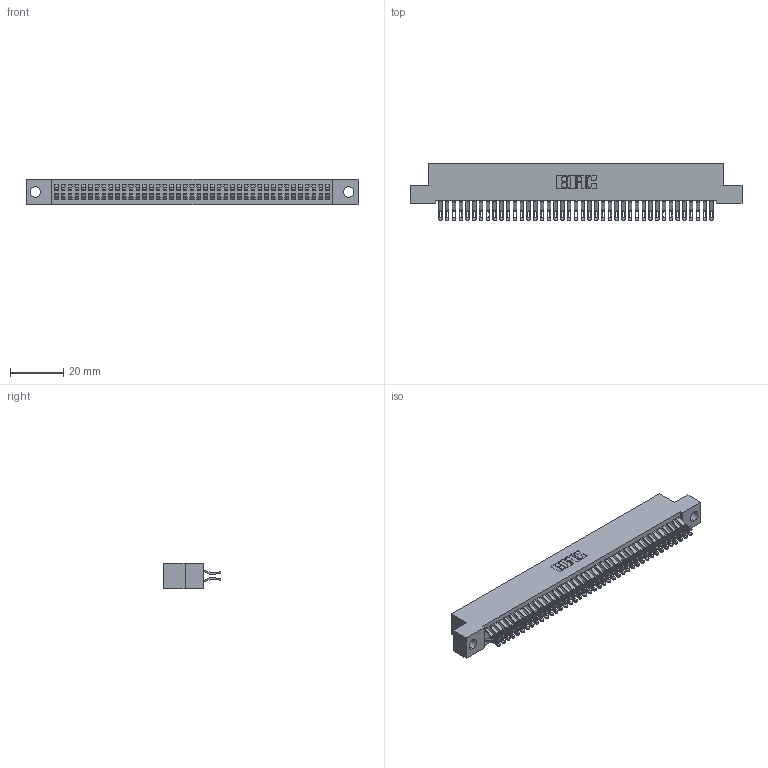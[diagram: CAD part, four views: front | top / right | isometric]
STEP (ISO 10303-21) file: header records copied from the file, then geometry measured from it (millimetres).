
FILE_DESCRIPTION (( 'STEP AP203' ), '1' );
FILE_NAME ('342-082-555-204.STEP', '2018-08-13T16:43:35', ( '' ), ( '' ), 'SwSTEP 2.0', 'SolidWorks 2016', '' );
FILE_SCHEMA (( 'CONFIG_CONTROL_DESIGN' ));
Length unit declared in the file: inch
Products named in the file (3): 342 Part_.156 TH; 345-292-001_555 Tail; 342-082-555-204
Assembly tree (83 placements, depth 2):
  342-082-555-204
    342 Part_.156 TH
    345-292-001_555 Tail  x82
Bounding box: 124.46 x 21.47 x 9.4 mm (x, y, z)
Volume: 11318.8 mm3; surface area: 19017.2 mm2
Topology: 83 solids, 83 shells, 4866 faces, 15305 edges, 10202 vertices
Faces by surface type: plane 2854, cylinder 2012
Entity records: 26703 total; most frequent: CARTESIAN_POINT 4460, ORIENTED_EDGE 4366, DIRECTION 3783, EDGE_CURVE 2183, VECTOR 2035, LINE 2035, VERTEX_POINT 1454, AXIS2_PLACEMENT_3D 874
